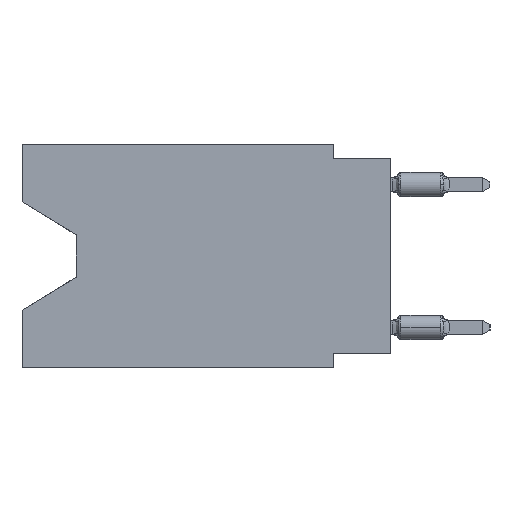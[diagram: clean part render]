
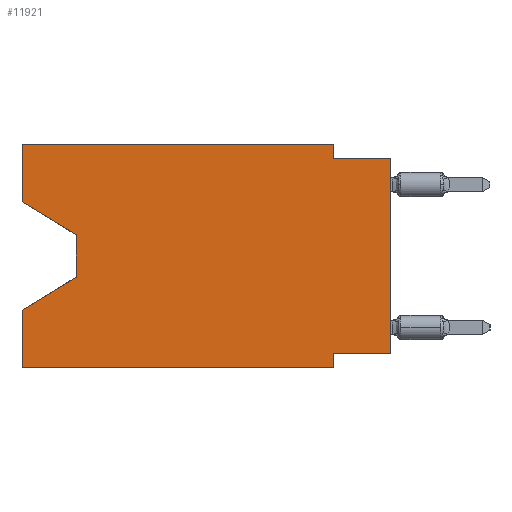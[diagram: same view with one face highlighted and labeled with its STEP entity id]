
A CAD part, left-side view. The second image highlights one B-rep face of the part: STEP entity #11921.
In plain terms, the highlighted planar face has unit normal (-1, 0, 0).
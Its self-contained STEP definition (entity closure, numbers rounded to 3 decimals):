
#1242 = AXIS2_PLACEMENT_3D ( 'NONE', #29353, #25922, #21442 ) ;
#1859 = LINE ( 'NONE', #49693, #2383 ) ;
#2297 = EDGE_CURVE ( 'NONE', #41015, #13871, #29237, .T. ) ;
#2383 = VECTOR ( 'NONE', #22488, 1000. ) ;
#2415 = VERTEX_POINT ( 'NONE', #14671 ) ;
#2489 = EDGE_LOOP ( 'NONE', ( #38468, #51310, #22024, #19574, #51220, #30167, #32601, #38335, #7019, #27820, #3689, #17716 ) ) ;
#3263 = EDGE_CURVE ( 'NONE', #2415, #45943, #1859, .T. ) ;
#3689 = ORIENTED_EDGE ( 'NONE', *, *, #33964, .F. ) ;
#3713 = CARTESIAN_POINT ( 'NONE',  ( 0., 13.97, -4.013 ) ) ;
#4342 = CARTESIAN_POINT ( 'NONE',  ( 0., 0., 0. ) ) ;
#4749 = VECTOR ( 'NONE', #7678, 1000. ) ;
#5111 = VECTOR ( 'NONE', #28374, 1000. ) ;
#5310 = FACE_OUTER_BOUND ( 'NONE', #2489, .T. ) ;
#6542 = LINE ( 'NONE', #10248, #46983 ) ;
#7019 = ORIENTED_EDGE ( 'NONE', *, *, #36480, .F. ) ;
#7506 = DIRECTION ( 'NONE',  ( 0., 0., 1. ) ) ;
#7678 = DIRECTION ( 'NONE',  ( 0., 0., -1. ) ) ;
#8064 = CARTESIAN_POINT ( 'NONE',  ( 0., 0., -9.271 ) ) ;
#8461 = VECTOR ( 'NONE', #49568, 1000. ) ;
#8568 = DIRECTION ( 'NONE',  ( 0., 0., 1. ) ) ;
#9190 = CARTESIAN_POINT ( 'NONE',  ( 0., 2.54, -9.906 ) ) ;
#9221 = LINE ( 'NONE', #33255, #43247 ) ;
#10248 = CARTESIAN_POINT ( 'NONE',  ( 0., 16.383, 0. ) ) ;
#10488 = VECTOR ( 'NONE', #8568, 1000. ) ;
#10497 = DIRECTION ( 'NONE',  ( 0., 0., 1. ) ) ;
#11777 = DIRECTION ( 'NONE',  ( 0., -1., 0. ) ) ;
#11921 = ADVANCED_FACE ( 'NONE', ( #5310 ), #45715, .F. ) ;
#12074 = VECTOR ( 'NONE', #44424, 1000. ) ;
#13871 = VERTEX_POINT ( 'NONE', #9190 ) ;
#14630 = EDGE_CURVE ( 'NONE', #32891, #25027, #28898, .T. ) ;
#14671 = CARTESIAN_POINT ( 'NONE',  ( 0., 2.54, 0. ) ) ;
#15009 = VERTEX_POINT ( 'NONE', #26988 ) ;
#15178 = LINE ( 'NONE', #31270, #23487 ) ;
#17091 = CARTESIAN_POINT ( 'NONE',  ( 0., 2.54, -9.906 ) ) ;
#17716 = ORIENTED_EDGE ( 'NONE', *, *, #31447, .F. ) ;
#19257 = EDGE_CURVE ( 'NONE', #15009, #30871, #41999, .T. ) ;
#19574 = ORIENTED_EDGE ( 'NONE', *, *, #30090, .F. ) ;
#21442 = DIRECTION ( 'NONE',  ( 0., 0., -1. ) ) ;
#22024 = ORIENTED_EDGE ( 'NONE', *, *, #45224, .T. ) ;
#22213 = CARTESIAN_POINT ( 'NONE',  ( 0., 16.383, -7.36 ) ) ;
#22488 = DIRECTION ( 'NONE',  ( 0., 0., -1. ) ) ;
#23301 = VERTEX_POINT ( 'NONE', #33792 ) ;
#23487 = VECTOR ( 'NONE', #7506, 1000. ) ;
#23588 = LINE ( 'NONE', #47066, #40047 ) ;
#24387 = VERTEX_POINT ( 'NONE', #22213 ) ;
#24739 = EDGE_CURVE ( 'NONE', #47097, #13871, #9221, .T. ) ;
#25027 = VERTEX_POINT ( 'NONE', #51994 ) ;
#25320 = VECTOR ( 'NONE', #11777, 1000. ) ;
#25922 = DIRECTION ( 'NONE',  ( 1., 0., 0. ) ) ;
#26726 = VERTEX_POINT ( 'NONE', #28679 ) ;
#26988 = CARTESIAN_POINT ( 'NONE',  ( 0., 16.383, -2.546 ) ) ;
#27820 = ORIENTED_EDGE ( 'NONE', *, *, #3263, .F. ) ;
#28374 = DIRECTION ( 'NONE',  ( 0., -0.855, -0.519 ) ) ;
#28679 = CARTESIAN_POINT ( 'NONE',  ( 0., 13.97, -5.893 ) ) ;
#28898 = LINE ( 'NONE', #4342, #10488 ) ;
#29237 = LINE ( 'NONE', #17091, #8461 ) ;
#29353 = CARTESIAN_POINT ( 'NONE',  ( 0., 16.383, 0. ) ) ;
#29585 = CARTESIAN_POINT ( 'NONE',  ( 0., 16.383, -2.546 ) ) ;
#30090 = EDGE_CURVE ( 'NONE', #47097, #24387, #6542, .T. ) ;
#30167 = ORIENTED_EDGE ( 'NONE', *, *, #2297, .F. ) ;
#30871 = VERTEX_POINT ( 'NONE', #42527 ) ;
#31270 = CARTESIAN_POINT ( 'NONE',  ( 0., 16.383, 0. ) ) ;
#31447 = EDGE_CURVE ( 'NONE', #15009, #23301, #15178, .T. ) ;
#32601 = ORIENTED_EDGE ( 'NONE', *, *, #35355, .F. ) ;
#32891 = VERTEX_POINT ( 'NONE', #8064 ) ;
#33008 = CARTESIAN_POINT ( 'NONE',  ( 0., 2.54, -9.271 ) ) ;
#33152 = CARTESIAN_POINT ( 'NONE',  ( 0., 0., -9.271 ) ) ;
#33255 = CARTESIAN_POINT ( 'NONE',  ( 0., 16.383, -9.906 ) ) ;
#33792 = CARTESIAN_POINT ( 'NONE',  ( 0., 16.383, 0. ) ) ;
#33964 = EDGE_CURVE ( 'NONE', #23301, #2415, #47681, .T. ) ;
#34565 = VECTOR ( 'NONE', #39147, 1000. ) ;
#35355 = EDGE_CURVE ( 'NONE', #32891, #41015, #40318, .T. ) ;
#35432 = CARTESIAN_POINT ( 'NONE',  ( 0., 0., -0.635 ) ) ;
#36480 = EDGE_CURVE ( 'NONE', #45943, #25027, #43082, .T. ) ;
#38254 = CARTESIAN_POINT ( 'NONE',  ( 0., 16.383, -9.906 ) ) ;
#38335 = ORIENTED_EDGE ( 'NONE', *, *, #14630, .T. ) ;
#38468 = ORIENTED_EDGE ( 'NONE', *, *, #19257, .T. ) ;
#39147 = DIRECTION ( 'NONE',  ( 0., 1., 0. ) ) ;
#40047 = VECTOR ( 'NONE', #47327, 1000. ) ;
#40318 = LINE ( 'NONE', #33152, #34565 ) ;
#41015 = VERTEX_POINT ( 'NONE', #33008 ) ;
#41999 = LINE ( 'NONE', #29585, #5111 ) ;
#42089 = EDGE_CURVE ( 'NONE', #30871, #26726, #43597, .T. ) ;
#42468 = CARTESIAN_POINT ( 'NONE',  ( 0., 2.54, -0.635 ) ) ;
#42527 = CARTESIAN_POINT ( 'NONE',  ( 0., 13.97, -4.013 ) ) ;
#43082 = LINE ( 'NONE', #35432, #12074 ) ;
#43247 = VECTOR ( 'NONE', #48869, 1000. ) ;
#43597 = LINE ( 'NONE', #3713, #4749 ) ;
#44424 = DIRECTION ( 'NONE',  ( 0., -1., 0. ) ) ;
#45224 = EDGE_CURVE ( 'NONE', #26726, #24387, #23588, .T. ) ;
#45715 = PLANE ( 'NONE',  #1242 ) ;
#45943 = VERTEX_POINT ( 'NONE', #42468 ) ;
#46983 = VECTOR ( 'NONE', #10497, 1000. ) ;
#47066 = CARTESIAN_POINT ( 'NONE',  ( 0., 13.97, -5.893 ) ) ;
#47097 = VERTEX_POINT ( 'NONE', #38254 ) ;
#47327 = DIRECTION ( 'NONE',  ( 0., 0.855, -0.519 ) ) ;
#47681 = LINE ( 'NONE', #47952, #25320 ) ;
#47952 = CARTESIAN_POINT ( 'NONE',  ( 0., 16.383, 0. ) ) ;
#48869 = DIRECTION ( 'NONE',  ( 0., -1., 0. ) ) ;
#49568 = DIRECTION ( 'NONE',  ( 0., 0., -1. ) ) ;
#49693 = CARTESIAN_POINT ( 'NONE',  ( 0., 2.54, 0. ) ) ;
#51220 = ORIENTED_EDGE ( 'NONE', *, *, #24739, .T. ) ;
#51310 = ORIENTED_EDGE ( 'NONE', *, *, #42089, .T. ) ;
#51994 = CARTESIAN_POINT ( 'NONE',  ( 0., 0., -0.635 ) ) ;
